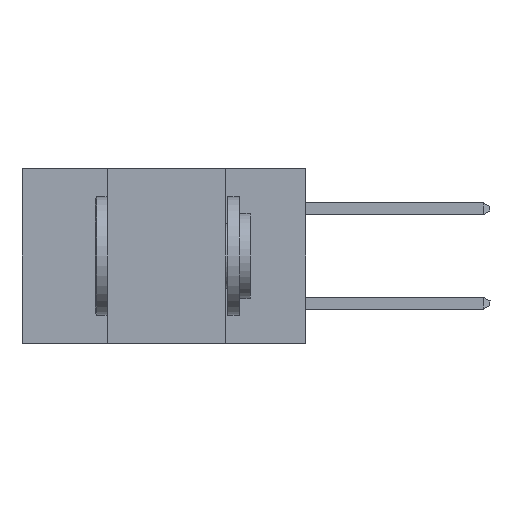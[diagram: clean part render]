
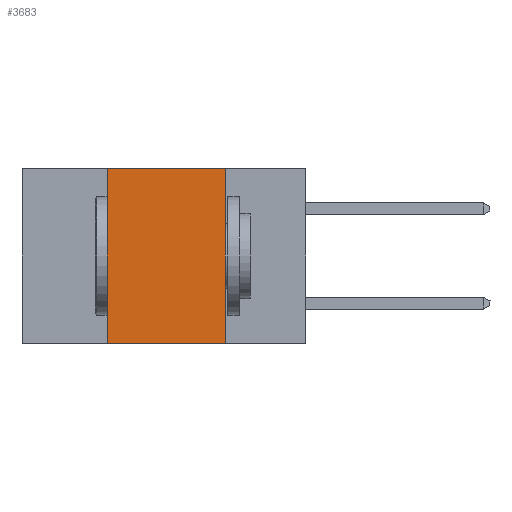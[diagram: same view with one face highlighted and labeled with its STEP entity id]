
A CAD part, left-side view. The second image highlights one B-rep face of the part: STEP entity #3683.
In plain terms, the highlighted planar face has unit normal (-1, 0, 0).
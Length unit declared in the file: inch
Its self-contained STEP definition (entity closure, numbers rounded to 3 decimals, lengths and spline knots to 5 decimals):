
#791 = DIRECTION ( 'NONE',  ( 0., 0., 1. ) ) ;
#1026 = LINE ( 'NONE', #15593, #14661 ) ;
#1192 = VECTOR ( 'NONE', #10174, 39.37008 ) ;
#1417 = CARTESIAN_POINT ( 'NONE',  ( 0., 0.6, 0. ) ) ;
#1505 = CARTESIAN_POINT ( 'NONE',  ( 0., 0.6, 0. ) ) ;
#1699 = DIRECTION ( 'NONE',  ( 0., 0., -1. ) ) ;
#1827 = ORIENTED_EDGE ( 'NONE', *, *, #11701, .F. ) ;
#2788 = EDGE_CURVE ( 'NONE', #8779, #9826, #15349, .T. ) ;
#2899 = DIRECTION ( 'NONE',  ( 0., -1., 0. ) ) ;
#3683 = ADVANCED_FACE ( 'NONE', ( #9295 ), #5882, .F. ) ;
#4277 = VECTOR ( 'NONE', #791, 39.37008 ) ;
#4928 = CARTESIAN_POINT ( 'NONE',  ( 0., 0.42, 0. ) ) ;
#5452 = CARTESIAN_POINT ( 'NONE',  ( 0., 0.17, 0. ) ) ;
#5882 = PLANE ( 'NONE',  #11227 ) ;
#6094 = EDGE_LOOP ( 'NONE', ( #9716, #1827, #6453, #17356 ) ) ;
#6104 = VERTEX_POINT ( 'NONE', #15790 ) ;
#6453 = ORIENTED_EDGE ( 'NONE', *, *, #15295, .F. ) ;
#8042 = LINE ( 'NONE', #4928, #4277 ) ;
#8779 = VERTEX_POINT ( 'NONE', #9658 ) ;
#9295 = FACE_OUTER_BOUND ( 'NONE', #6094, .T. ) ;
#9658 = CARTESIAN_POINT ( 'NONE',  ( 0., 0.42, -0.37 ) ) ;
#9716 = ORIENTED_EDGE ( 'NONE', *, *, #17583, .F. ) ;
#9826 = VERTEX_POINT ( 'NONE', #17260 ) ;
#10135 = LINE ( 'NONE', #1417, #1192 ) ;
#10174 = DIRECTION ( 'NONE',  ( 0., -1., 0. ) ) ;
#10696 = VECTOR ( 'NONE', #2899, 39.37008 ) ;
#11227 = AXIS2_PLACEMENT_3D ( 'NONE', #1505, #14359, #1699 ) ;
#11444 = CARTESIAN_POINT ( 'NONE',  ( 0., 0.6, -0.37 ) ) ;
#11701 = EDGE_CURVE ( 'NONE', #6104, #16184, #10135, .T. ) ;
#14359 = DIRECTION ( 'NONE',  ( 1., 0., 0. ) ) ;
#14661 = VECTOR ( 'NONE', #16975, 39.37008 ) ;
#15295 = EDGE_CURVE ( 'NONE', #8779, #6104, #8042, .T. ) ;
#15349 = LINE ( 'NONE', #11444, #10696 ) ;
#15593 = CARTESIAN_POINT ( 'NONE',  ( 0., 0.17, 0. ) ) ;
#15790 = CARTESIAN_POINT ( 'NONE',  ( 0., 0.42, 0. ) ) ;
#16184 = VERTEX_POINT ( 'NONE', #5452 ) ;
#16975 = DIRECTION ( 'NONE',  ( 0., 0., -1. ) ) ;
#17260 = CARTESIAN_POINT ( 'NONE',  ( 0., 0.17, -0.37 ) ) ;
#17356 = ORIENTED_EDGE ( 'NONE', *, *, #2788, .T. ) ;
#17583 = EDGE_CURVE ( 'NONE', #16184, #9826, #1026, .T. ) ;
